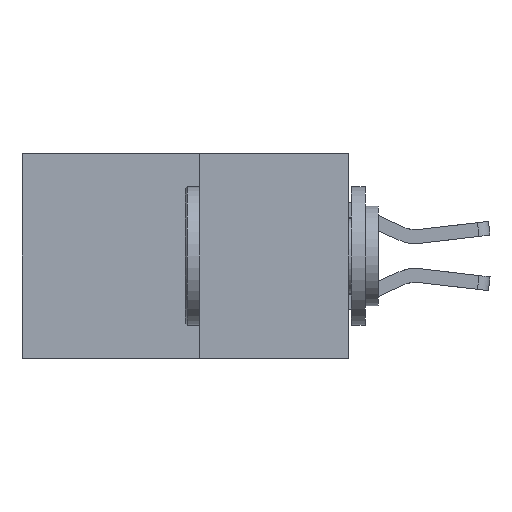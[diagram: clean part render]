
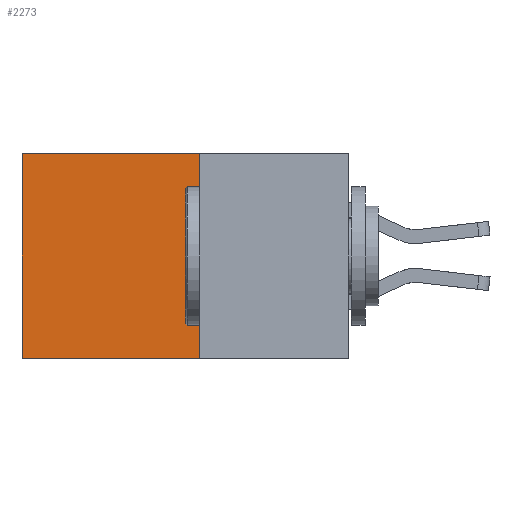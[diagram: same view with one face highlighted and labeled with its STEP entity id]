
A CAD part, left-side view. The second image highlights one B-rep face of the part: STEP entity #2273.
In plain terms, the highlighted planar face has unit normal (-1, 0, 0).
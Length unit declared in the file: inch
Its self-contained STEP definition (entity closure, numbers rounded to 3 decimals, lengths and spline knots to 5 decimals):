
#291 = VERTEX_POINT ( 'NONE', #2774 ) ;
#322 = VECTOR ( 'NONE', #9761, 39.37008 ) ;
#749 = CARTESIAN_POINT ( 'NONE',  ( 0.277, 0.27, -0.37 ) ) ;
#1146 = VECTOR ( 'NONE', #2707, 39.37008 ) ;
#1260 = CARTESIAN_POINT ( 'NONE',  ( 0.277, 0.59, -0.37 ) ) ;
#1482 = ORIENTED_EDGE ( 'NONE', *, *, #9362, .T. ) ;
#1515 = ORIENTED_EDGE ( 'NONE', *, *, #8050, .F. ) ;
#1544 = ORIENTED_EDGE ( 'NONE', *, *, #6774, .F. ) ;
#1600 = ORIENTED_EDGE ( 'NONE', *, *, #8717, .T. ) ;
#2052 = CARTESIAN_POINT ( 'NONE',  ( 0.277, 0.27, -0.37 ) ) ;
#2109 = EDGE_LOOP ( 'NONE', ( #1600, #1544, #1515, #1482 ) ) ;
#2128 = CARTESIAN_POINT ( 'NONE',  ( 0.277, 0.27, 0. ) ) ;
#2273 = ADVANCED_FACE ( 'NONE', ( #6511 ), #9520, .F. ) ;
#2486 = LINE ( 'NONE', #4599, #322 ) ;
#2707 = DIRECTION ( 'NONE',  ( 0., 1., 0. ) ) ;
#2774 = CARTESIAN_POINT ( 'NONE',  ( 0.277, 0.59, -0.37 ) ) ;
#2905 = DIRECTION ( 'NONE',  ( 0., 0., -1. ) ) ;
#3247 = LINE ( 'NONE', #8490, #1146 ) ;
#3296 = CARTESIAN_POINT ( 'NONE',  ( 0.277, 0.27, -0.37 ) ) ;
#3395 = VERTEX_POINT ( 'NONE', #3296 ) ;
#3707 = LINE ( 'NONE', #1260, #9341 ) ;
#3955 = VECTOR ( 'NONE', #4292, 39.37008 ) ;
#4292 = DIRECTION ( 'NONE',  ( 0., 1., 0. ) ) ;
#4599 = CARTESIAN_POINT ( 'NONE',  ( 0.277, 0.27, -0.37 ) ) ;
#5654 = DIRECTION ( 'NONE',  ( 0., 0., -1. ) ) ;
#5754 = DIRECTION ( 'NONE',  ( 1., 0., 0. ) ) ;
#5794 = VERTEX_POINT ( 'NONE', #8287 ) ;
#5919 = LINE ( 'NONE', #2052, #3955 ) ;
#6511 = FACE_OUTER_BOUND ( 'NONE', #2109, .T. ) ;
#6774 = EDGE_CURVE ( 'NONE', #3395, #291, #5919, .T. ) ;
#6848 = VERTEX_POINT ( 'NONE', #2128 ) ;
#8050 = EDGE_CURVE ( 'NONE', #6848, #3395, #2486, .T. ) ;
#8209 = AXIS2_PLACEMENT_3D ( 'NONE', #749, #5754, #5654 ) ;
#8287 = CARTESIAN_POINT ( 'NONE',  ( 0.277, 0.59, 0. ) ) ;
#8490 = CARTESIAN_POINT ( 'NONE',  ( 0.277, 0.27, 0. ) ) ;
#8717 = EDGE_CURVE ( 'NONE', #5794, #291, #3707, .T. ) ;
#9341 = VECTOR ( 'NONE', #2905, 39.37008 ) ;
#9362 = EDGE_CURVE ( 'NONE', #6848, #5794, #3247, .T. ) ;
#9520 = PLANE ( 'NONE',  #8209 ) ;
#9761 = DIRECTION ( 'NONE',  ( 0., 0., -1. ) ) ;
